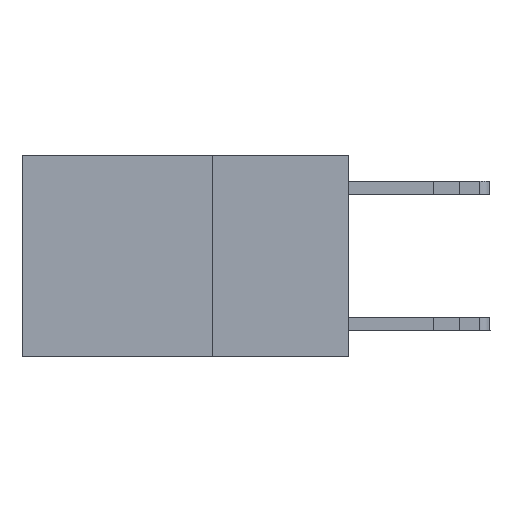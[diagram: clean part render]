
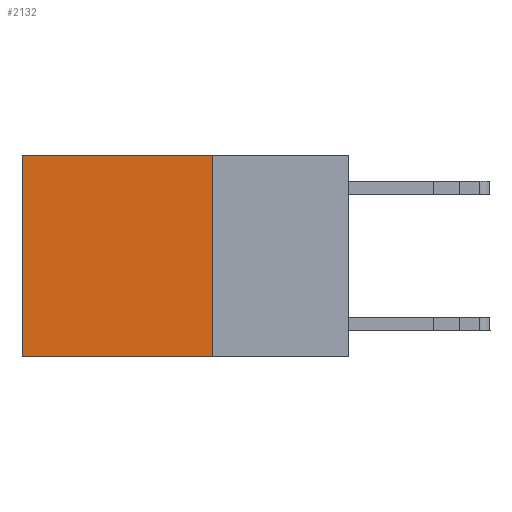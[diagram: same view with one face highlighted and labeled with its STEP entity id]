
A CAD part, left-side view. The second image highlights one B-rep face of the part: STEP entity #2132.
In plain terms, the highlighted planar face has unit normal (-1, 0, 0).
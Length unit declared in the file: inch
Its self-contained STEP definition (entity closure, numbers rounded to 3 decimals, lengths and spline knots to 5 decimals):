
#793 = CARTESIAN_POINT ( 'NONE',  ( 0.2625, 0.25, -0.37 ) ) ;
#1218 = LINE ( 'NONE', #2970, #8587 ) ;
#1373 = CARTESIAN_POINT ( 'NONE',  ( 0.2625, 0.25, 0. ) ) ;
#1390 = ORIENTED_EDGE ( 'NONE', *, *, #6291, .T. ) ;
#2012 = DIRECTION ( 'NONE',  ( 0., 0., -1. ) ) ;
#2132 = ADVANCED_FACE ( 'NONE', ( #11420 ), #10364, .F. ) ;
#2162 = CARTESIAN_POINT ( 'NONE',  ( 0.2625, 0.25, 0. ) ) ;
#2217 = CARTESIAN_POINT ( 'NONE',  ( 0.2625, 0.25, 0. ) ) ;
#2628 = EDGE_CURVE ( 'NONE', #5529, #10940, #1218, .T. ) ;
#2633 = CARTESIAN_POINT ( 'NONE',  ( 0.2625, 0.6, 0. ) ) ;
#2807 = ORIENTED_EDGE ( 'NONE', *, *, #5216, .F. ) ;
#2970 = CARTESIAN_POINT ( 'NONE',  ( 0.2625, 0.6, 0. ) ) ;
#4192 = ORIENTED_EDGE ( 'NONE', *, *, #2628, .T. ) ;
#4369 = EDGE_LOOP ( 'NONE', ( #4192, #11295, #2807, #1390 ) ) ;
#5216 = EDGE_CURVE ( 'NONE', #7999, #10577, #11057, .T. ) ;
#5469 = CARTESIAN_POINT ( 'NONE',  ( 0.2625, 0.25, -0.37 ) ) ;
#5529 = VERTEX_POINT ( 'NONE', #2633 ) ;
#5637 = VECTOR ( 'NONE', #2012, 39.37008 ) ;
#5774 = AXIS2_PLACEMENT_3D ( 'NONE', #2162, #9656, #8601 ) ;
#6210 = CARTESIAN_POINT ( 'NONE',  ( 0.2625, 0.6, -0.37 ) ) ;
#6291 = EDGE_CURVE ( 'NONE', #7999, #5529, #7947, .T. ) ;
#6594 = CARTESIAN_POINT ( 'NONE',  ( 0.2625, 0.25, 0. ) ) ;
#7104 = LINE ( 'NONE', #793, #7399 ) ;
#7201 = DIRECTION ( 'NONE',  ( 0., 1., 0. ) ) ;
#7399 = VECTOR ( 'NONE', #7201, 39.37008 ) ;
#7947 = LINE ( 'NONE', #2217, #9875 ) ;
#7999 = VERTEX_POINT ( 'NONE', #1373 ) ;
#8068 = DIRECTION ( 'NONE',  ( 0., 1., 0. ) ) ;
#8587 = VECTOR ( 'NONE', #10105, 39.37008 ) ;
#8601 = DIRECTION ( 'NONE',  ( 0., 0., -1. ) ) ;
#9656 = DIRECTION ( 'NONE',  ( 1., 0., 0. ) ) ;
#9875 = VECTOR ( 'NONE', #8068, 39.37008 ) ;
#10105 = DIRECTION ( 'NONE',  ( 0., 0., -1. ) ) ;
#10364 = PLANE ( 'NONE',  #5774 ) ;
#10577 = VERTEX_POINT ( 'NONE', #5469 ) ;
#10578 = EDGE_CURVE ( 'NONE', #10577, #10940, #7104, .T. ) ;
#10940 = VERTEX_POINT ( 'NONE', #6210 ) ;
#11057 = LINE ( 'NONE', #6594, #5637 ) ;
#11295 = ORIENTED_EDGE ( 'NONE', *, *, #10578, .F. ) ;
#11420 = FACE_OUTER_BOUND ( 'NONE', #4369, .T. ) ;
